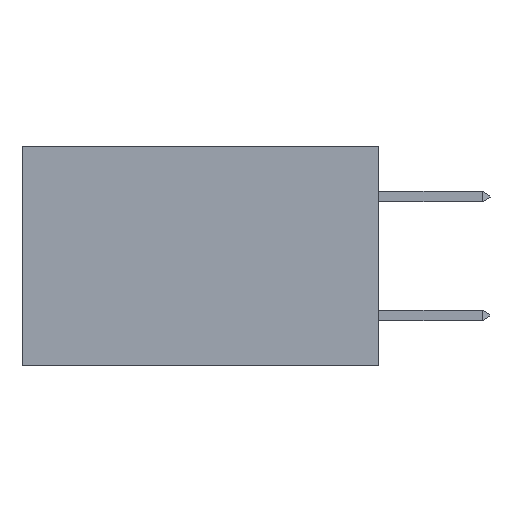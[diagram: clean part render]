
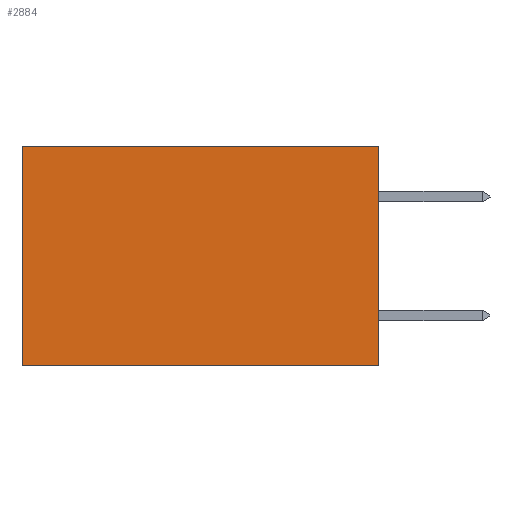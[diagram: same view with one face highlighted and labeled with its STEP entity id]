
A CAD part, left-side view. The second image highlights one B-rep face of the part: STEP entity #2884.
In plain terms, the highlighted planar face has unit normal (-1, 0, 0).
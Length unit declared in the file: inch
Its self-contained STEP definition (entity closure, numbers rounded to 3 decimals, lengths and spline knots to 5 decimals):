
#693 = VERTEX_POINT ( 'NONE', #17758 ) ;
#999 = EDGE_CURVE ( 'NONE', #14308, #693, #5051, .T. ) ;
#1698 = LINE ( 'NONE', #16896, #16710 ) ;
#2054 = ORIENTED_EDGE ( 'NONE', *, *, #10732, .F. ) ;
#2847 = ORIENTED_EDGE ( 'NONE', *, *, #12384, .F. ) ;
#2884 = ADVANCED_FACE ( 'NONE', ( #16023 ), #3633, .F. ) ;
#3590 = DIRECTION ( 'NONE',  ( 0., 0., -1. ) ) ;
#3633 = PLANE ( 'NONE',  #6873 ) ;
#3671 = CARTESIAN_POINT ( 'NONE',  ( 0.298, 0.6, 0. ) ) ;
#4363 = DIRECTION ( 'NONE',  ( 1., 0., 0. ) ) ;
#4378 = CARTESIAN_POINT ( 'NONE',  ( 0.298, 0., 0. ) ) ;
#4725 = LINE ( 'NONE', #12704, #15998 ) ;
#5051 = LINE ( 'NONE', #3671, #8850 ) ;
#6006 = EDGE_CURVE ( 'NONE', #10462, #14308, #15354, .T. ) ;
#6873 = AXIS2_PLACEMENT_3D ( 'NONE', #4378, #4363, #18183 ) ;
#7172 = EDGE_LOOP ( 'NONE', ( #8779, #2054, #2847, #13342 ) ) ;
#8302 = VECTOR ( 'NONE', #9663, 39.37008 ) ;
#8405 = VERTEX_POINT ( 'NONE', #10961 ) ;
#8779 = ORIENTED_EDGE ( 'NONE', *, *, #999, .T. ) ;
#8850 = VECTOR ( 'NONE', #3590, 39.37008 ) ;
#9663 = DIRECTION ( 'NONE',  ( 0., 1., 0. ) ) ;
#10462 = VERTEX_POINT ( 'NONE', #10825 ) ;
#10732 = EDGE_CURVE ( 'NONE', #8405, #693, #1698, .T. ) ;
#10825 = CARTESIAN_POINT ( 'NONE',  ( 0.298, 0., 0. ) ) ;
#10961 = CARTESIAN_POINT ( 'NONE',  ( 0.298, 0., -0.37 ) ) ;
#12378 = DIRECTION ( 'NONE',  ( 0., 1., 0. ) ) ;
#12384 = EDGE_CURVE ( 'NONE', #10462, #8405, #4725, .T. ) ;
#12704 = CARTESIAN_POINT ( 'NONE',  ( 0.298, 0., 0. ) ) ;
#13342 = ORIENTED_EDGE ( 'NONE', *, *, #6006, .T. ) ;
#14002 = DIRECTION ( 'NONE',  ( 0., 0., -1. ) ) ;
#14127 = CARTESIAN_POINT ( 'NONE',  ( 0.298, 0.6, 0. ) ) ;
#14308 = VERTEX_POINT ( 'NONE', #14127 ) ;
#15354 = LINE ( 'NONE', #16625, #8302 ) ;
#15998 = VECTOR ( 'NONE', #14002, 39.37008 ) ;
#16023 = FACE_OUTER_BOUND ( 'NONE', #7172, .T. ) ;
#16625 = CARTESIAN_POINT ( 'NONE',  ( 0.298, 0., 0. ) ) ;
#16710 = VECTOR ( 'NONE', #12378, 39.37008 ) ;
#16896 = CARTESIAN_POINT ( 'NONE',  ( 0.298, 0., -0.37 ) ) ;
#17758 = CARTESIAN_POINT ( 'NONE',  ( 0.298, 0.6, -0.37 ) ) ;
#18183 = DIRECTION ( 'NONE',  ( 0., 0., -1. ) ) ;
